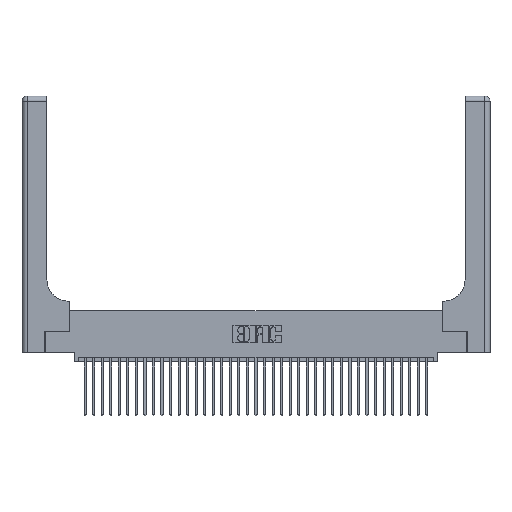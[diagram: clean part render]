
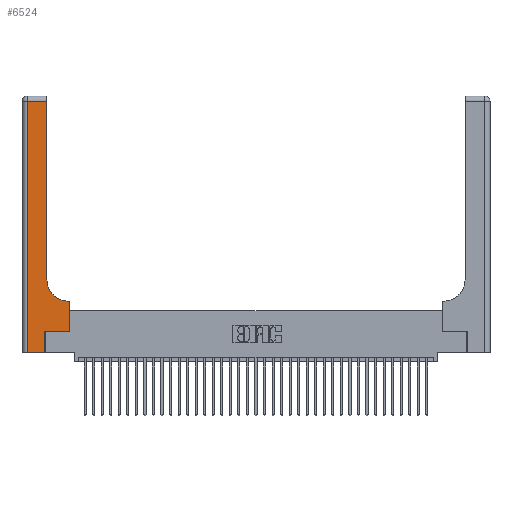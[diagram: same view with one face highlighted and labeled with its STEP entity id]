
A CAD part, top view. The second image highlights one B-rep face of the part: STEP entity #6524.
In plain terms, the highlighted planar face has unit normal (0, 0, 1).
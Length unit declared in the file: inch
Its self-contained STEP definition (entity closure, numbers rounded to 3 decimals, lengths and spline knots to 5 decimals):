
#511 = CARTESIAN_POINT ( 'NONE',  ( 0.06, 3., 0.37 ) ) ;
#1401 = CARTESIAN_POINT ( 'NONE',  ( 0.5415, 0.85, 0.37 ) ) ;
#2250 = CARTESIAN_POINT ( 'NONE',  ( 0.2915, 0.85, 0.37 ) ) ;
#2286 = CARTESIAN_POINT ( 'NONE',  ( 0.5585, 0.6, 0.37 ) ) ;
#3507 = DIRECTION ( 'NONE',  ( 0., -1., 0. ) ) ;
#4326 = VERTEX_POINT ( 'NONE', #6132 ) ;
#4357 = DIRECTION ( 'NONE',  ( 1., 0., 0. ) ) ;
#5496 = LINE ( 'NONE', #11568, #26847 ) ;
#6132 = CARTESIAN_POINT ( 'NONE',  ( 0.06, 0., 0.37 ) ) ;
#6454 = LINE ( 'NONE', #11225, #27797 ) ;
#6524 = ADVANCED_FACE ( 'NONE', ( #14219 ), #11097, .F. ) ;
#6573 = EDGE_CURVE ( 'NONE', #25033, #14246, #6454, .T. ) ;
#7007 = EDGE_CURVE ( 'NONE', #4326, #20069, #8262, .T. ) ;
#8262 = LINE ( 'NONE', #19338, #30464 ) ;
#8901 = VECTOR ( 'NONE', #33662, 39.37008 ) ;
#10687 = DIRECTION ( 'NONE',  ( 1., 0., 0. ) ) ;
#11097 = PLANE ( 'NONE',  #20934 ) ;
#11225 = CARTESIAN_POINT ( 'NONE',  ( 0.269, 0.25, 0.37 ) ) ;
#11555 = VECTOR ( 'NONE', #3507, 39.37008 ) ;
#11568 = CARTESIAN_POINT ( 'NONE',  ( 0.2915, 0.6, 0.37 ) ) ;
#11581 = VECTOR ( 'NONE', #15860, 39.37008 ) ;
#12019 = AXIS2_PLACEMENT_3D ( 'NONE', #1401, #21775, #4357 ) ;
#12465 = LINE ( 'NONE', #511, #11555 ) ;
#12725 = VERTEX_POINT ( 'NONE', #2286 ) ;
#13294 = CARTESIAN_POINT ( 'NONE',  ( 0.06, 2.94, 0.37 ) ) ;
#13756 = VERTEX_POINT ( 'NONE', #33168 ) ;
#13918 = CARTESIAN_POINT ( 'NONE',  ( 0., 3., 0.37 ) ) ;
#14038 = DIRECTION ( 'NONE',  ( -1., 0., 0. ) ) ;
#14219 = FACE_OUTER_BOUND ( 'NONE', #34319, .T. ) ;
#14246 = VERTEX_POINT ( 'NONE', #29813 ) ;
#14645 = EDGE_CURVE ( 'NONE', #12725, #18735, #5496, .T. ) ;
#15332 = ORIENTED_EDGE ( 'NONE', *, *, #7007, .T. ) ;
#15609 = LINE ( 'NONE', #31984, #28263 ) ;
#15860 = DIRECTION ( 'NONE',  ( 0., 1., 0. ) ) ;
#17126 = ORIENTED_EDGE ( 'NONE', *, *, #26693, .T. ) ;
#17334 = ORIENTED_EDGE ( 'NONE', *, *, #20058, .T. ) ;
#17467 = VERTEX_POINT ( 'NONE', #2250 ) ;
#17554 = DIRECTION ( 'NONE',  ( 0., 1., 0. ) ) ;
#18250 = ORIENTED_EDGE ( 'NONE', *, *, #18986, .T. ) ;
#18735 = VERTEX_POINT ( 'NONE', #32185 ) ;
#18986 = EDGE_CURVE ( 'NONE', #17467, #13756, #19311, .T. ) ;
#19311 = LINE ( 'NONE', #35964, #11581 ) ;
#19338 = CARTESIAN_POINT ( 'NONE',  ( 0., 0., 0.37 ) ) ;
#19794 = ORIENTED_EDGE ( 'NONE', *, *, #22783, .T. ) ;
#20058 = EDGE_CURVE ( 'NONE', #20069, #25033, #15609, .T. ) ;
#20069 = VERTEX_POINT ( 'NONE', #34890 ) ;
#20350 = CARTESIAN_POINT ( 'NONE',  ( 0.269, 0.25, 0.37 ) ) ;
#20843 = LINE ( 'NONE', #27564, #35299 ) ;
#20934 = AXIS2_PLACEMENT_3D ( 'NONE', #13918, #31355, #14038 ) ;
#21775 = DIRECTION ( 'NONE',  ( 0., 0., -1. ) ) ;
#22069 = ORIENTED_EDGE ( 'NONE', *, *, #34331, .T. ) ;
#22783 = EDGE_CURVE ( 'NONE', #37286, #4326, #12465, .T. ) ;
#23335 = ORIENTED_EDGE ( 'NONE', *, *, #28292, .T. ) ;
#24357 = LINE ( 'NONE', #30750, #8901 ) ;
#25033 = VERTEX_POINT ( 'NONE', #20350 ) ;
#25705 = DIRECTION ( 'NONE',  ( 1., 0., 0. ) ) ;
#26693 = EDGE_CURVE ( 'NONE', #18735, #17467, #32614, .T. ) ;
#26847 = VECTOR ( 'NONE', #31823, 39.37008 ) ;
#27564 = CARTESIAN_POINT ( 'NONE',  ( 0., 2.94, 0.37 ) ) ;
#27576 = ORIENTED_EDGE ( 'NONE', *, *, #14645, .T. ) ;
#27797 = VECTOR ( 'NONE', #25705, 39.37008 ) ;
#28263 = VECTOR ( 'NONE', #17554, 39.37008 ) ;
#28292 = EDGE_CURVE ( 'NONE', #14246, #12725, #24357, .T. ) ;
#29813 = CARTESIAN_POINT ( 'NONE',  ( 0.5585, 0.25, 0.37 ) ) ;
#30453 = DIRECTION ( 'NONE',  ( -1., 0., 0. ) ) ;
#30464 = VECTOR ( 'NONE', #10687, 39.37008 ) ;
#30750 = CARTESIAN_POINT ( 'NONE',  ( 0.5585, 0.25, 0.37 ) ) ;
#31355 = DIRECTION ( 'NONE',  ( 0., 0., -1. ) ) ;
#31823 = DIRECTION ( 'NONE',  ( -1., 0., 0. ) ) ;
#31984 = CARTESIAN_POINT ( 'NONE',  ( 0.269, 0., 0.37 ) ) ;
#32185 = CARTESIAN_POINT ( 'NONE',  ( 0.5415, 0.6, 0.37 ) ) ;
#32614 = CIRCLE ( 'NONE', #12019, 0.25 ) ;
#33147 = ORIENTED_EDGE ( 'NONE', *, *, #6573, .T. ) ;
#33168 = CARTESIAN_POINT ( 'NONE',  ( 0.2915, 2.94, 0.37 ) ) ;
#33662 = DIRECTION ( 'NONE',  ( 0., 1., 0. ) ) ;
#34319 = EDGE_LOOP ( 'NONE', ( #18250, #22069, #19794, #15332, #17334, #33147, #23335, #27576, #17126 ) ) ;
#34331 = EDGE_CURVE ( 'NONE', #13756, #37286, #20843, .T. ) ;
#34890 = CARTESIAN_POINT ( 'NONE',  ( 0.269, 0., 0.37 ) ) ;
#35299 = VECTOR ( 'NONE', #30453, 39.37008 ) ;
#35964 = CARTESIAN_POINT ( 'NONE',  ( 0.2915, 3., 0.37 ) ) ;
#37286 = VERTEX_POINT ( 'NONE', #13294 ) ;
